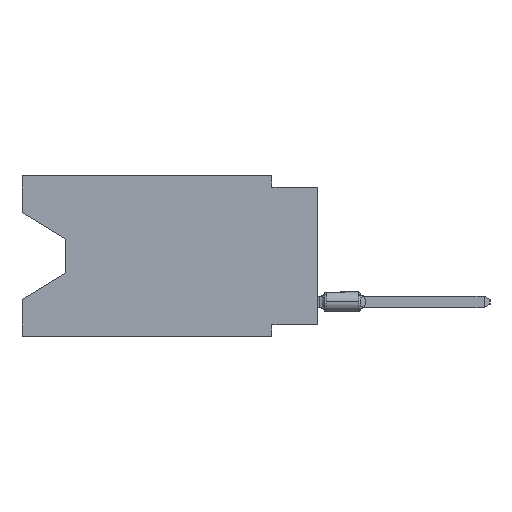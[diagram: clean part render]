
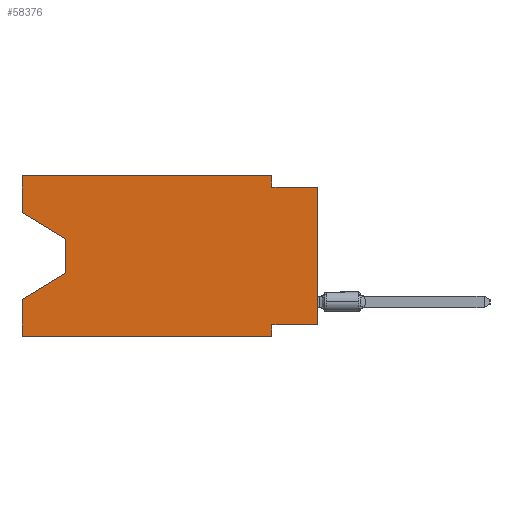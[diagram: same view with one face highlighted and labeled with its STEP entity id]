
A CAD part, left-side view. The second image highlights one B-rep face of the part: STEP entity #58376.
In plain terms, the highlighted planar face has unit normal (-1, 0, 0).
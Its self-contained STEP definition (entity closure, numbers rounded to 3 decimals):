
#305 = ORIENTED_EDGE ( 'NONE', *, *, #55115, .T. ) ;
#1327 = CARTESIAN_POINT ( 'NONE',  ( 0., 2.54, -8.89 ) ) ;
#1581 = DIRECTION ( 'NONE',  ( 0., -1., 0. ) ) ;
#2448 = CARTESIAN_POINT ( 'NONE',  ( 0., 16.383, -6.852 ) ) ;
#2837 = EDGE_CURVE ( 'NONE', #50765, #39058, #23167, .T. ) ;
#4071 = VERTEX_POINT ( 'NONE', #55797 ) ;
#4248 = LINE ( 'NONE', #29562, #50675 ) ;
#7455 = DIRECTION ( 'NONE',  ( 0., -0.855, -0.519 ) ) ;
#7603 = DIRECTION ( 'NONE',  ( 0., -1., 0. ) ) ;
#8316 = EDGE_CURVE ( 'NONE', #63367, #4071, #39837, .T. ) ;
#8692 = CARTESIAN_POINT ( 'NONE',  ( 0., 2.54, -0.635 ) ) ;
#9533 = VECTOR ( 'NONE', #29877, 1000. ) ;
#9950 = ORIENTED_EDGE ( 'NONE', *, *, #14065, .F. ) ;
#11351 = EDGE_CURVE ( 'NONE', #4071, #56030, #33874, .T. ) ;
#11638 = DIRECTION ( 'NONE',  ( 0., 0., 1. ) ) ;
#11701 = DIRECTION ( 'NONE',  ( 0., -1., 0. ) ) ;
#11794 = LINE ( 'NONE', #48024, #45046 ) ;
#12198 = ORIENTED_EDGE ( 'NONE', *, *, #36710, .F. ) ;
#14065 = EDGE_CURVE ( 'NONE', #38638, #59278, #53231, .T. ) ;
#14668 = DIRECTION ( 'NONE',  ( 1., 0., 0. ) ) ;
#14803 = LINE ( 'NONE', #50721, #9533 ) ;
#15726 = VECTOR ( 'NONE', #1581, 1000. ) ;
#16935 = CARTESIAN_POINT ( 'NONE',  ( 0., 2.54, -8.255 ) ) ;
#17046 = ORIENTED_EDGE ( 'NONE', *, *, #34735, .F. ) ;
#17070 = CARTESIAN_POINT ( 'NONE',  ( 0., 16.383, -2.038 ) ) ;
#18257 = VERTEX_POINT ( 'NONE', #30647 ) ;
#19648 = VERTEX_POINT ( 'NONE', #2448 ) ;
#19785 = PLANE ( 'NONE',  #64346 ) ;
#20865 = EDGE_CURVE ( 'NONE', #18257, #19648, #30411, .T. ) ;
#22042 = DIRECTION ( 'NONE',  ( 0., 0., -1. ) ) ;
#22312 = EDGE_LOOP ( 'NONE', ( #29484, #305, #37327, #27753, #54468, #50413, #12198, #62773, #9950, #17046, #22792, #58764 ) ) ;
#22792 = ORIENTED_EDGE ( 'NONE', *, *, #11351, .F. ) ;
#22970 = CARTESIAN_POINT ( 'NONE',  ( 0., 2.54, -8.89 ) ) ;
#23167 = LINE ( 'NONE', #1327, #33071 ) ;
#25918 = VECTOR ( 'NONE', #66521, 1000. ) ;
#26799 = EDGE_CURVE ( 'NONE', #63367, #64253, #28662, .T. ) ;
#27628 = DIRECTION ( 'NONE',  ( 0., 0., -1. ) ) ;
#27659 = VECTOR ( 'NONE', #11638, 1000. ) ;
#27753 = ORIENTED_EDGE ( 'NONE', *, *, #20865, .F. ) ;
#28565 = CARTESIAN_POINT ( 'NONE',  ( 0., 13.97, -3.505 ) ) ;
#28662 = LINE ( 'NONE', #17070, #35437 ) ;
#29390 = DIRECTION ( 'NONE',  ( 0., 0., 1. ) ) ;
#29484 = ORIENTED_EDGE ( 'NONE', *, *, #26799, .T. ) ;
#29562 = CARTESIAN_POINT ( 'NONE',  ( 0., 0., -8.255 ) ) ;
#29877 = DIRECTION ( 'NONE',  ( 0., 0., -1. ) ) ;
#30188 = EDGE_CURVE ( 'NONE', #64141, #59278, #32828, .T. ) ;
#30411 = LINE ( 'NONE', #67000, #44771 ) ;
#30419 = CARTESIAN_POINT ( 'NONE',  ( 0., 13.97, -5.385 ) ) ;
#30647 = CARTESIAN_POINT ( 'NONE',  ( 0., 16.383, -8.89 ) ) ;
#32828 = LINE ( 'NONE', #37625, #27659 ) ;
#33071 = VECTOR ( 'NONE', #49503, 1000. ) ;
#33281 = VECTOR ( 'NONE', #7603, 1000. ) ;
#33874 = LINE ( 'NONE', #59551, #55864 ) ;
#34735 = EDGE_CURVE ( 'NONE', #56030, #38638, #11794, .T. ) ;
#35385 = DIRECTION ( 'NONE',  ( 0., 1., 0. ) ) ;
#35437 = VECTOR ( 'NONE', #7455, 1000. ) ;
#36506 = EDGE_CURVE ( 'NONE', #18257, #39058, #59015, .T. ) ;
#36710 = EDGE_CURVE ( 'NONE', #64141, #50765, #4248, .T. ) ;
#37029 = VECTOR ( 'NONE', #43420, 1000. ) ;
#37327 = ORIENTED_EDGE ( 'NONE', *, *, #52037, .T. ) ;
#37625 = CARTESIAN_POINT ( 'NONE',  ( 0., 0., 0. ) ) ;
#38638 = VERTEX_POINT ( 'NONE', #8692 ) ;
#39058 = VERTEX_POINT ( 'NONE', #22970 ) ;
#39837 = LINE ( 'NONE', #40173, #25918 ) ;
#40173 = CARTESIAN_POINT ( 'NONE',  ( 0., 16.383, 0. ) ) ;
#40987 = FACE_OUTER_BOUND ( 'NONE', #22312, .T. ) ;
#43290 = CARTESIAN_POINT ( 'NONE',  ( 0., 16.383, -8.89 ) ) ;
#43420 = DIRECTION ( 'NONE',  ( 0., 0.855, -0.519 ) ) ;
#44771 = VECTOR ( 'NONE', #29390, 1000. ) ;
#45046 = VECTOR ( 'NONE', #22042, 1000. ) ;
#45323 = VERTEX_POINT ( 'NONE', #30419 ) ;
#48024 = CARTESIAN_POINT ( 'NONE',  ( 0., 2.54, 0. ) ) ;
#49503 = DIRECTION ( 'NONE',  ( 0., 0., -1. ) ) ;
#49918 = CARTESIAN_POINT ( 'NONE',  ( 0., 16.383, -2.038 ) ) ;
#50413 = ORIENTED_EDGE ( 'NONE', *, *, #2837, .F. ) ;
#50675 = VECTOR ( 'NONE', #35385, 1000. ) ;
#50721 = CARTESIAN_POINT ( 'NONE',  ( 0., 13.97, -3.505 ) ) ;
#50765 = VERTEX_POINT ( 'NONE', #16935 ) ;
#52037 = EDGE_CURVE ( 'NONE', #45323, #19648, #55023, .T. ) ;
#53231 = LINE ( 'NONE', #54455, #33281 ) ;
#54455 = CARTESIAN_POINT ( 'NONE',  ( 0., 0., -0.635 ) ) ;
#54468 = ORIENTED_EDGE ( 'NONE', *, *, #36506, .T. ) ;
#55023 = LINE ( 'NONE', #60503, #37029 ) ;
#55115 = EDGE_CURVE ( 'NONE', #64253, #45323, #14803, .T. ) ;
#55797 = CARTESIAN_POINT ( 'NONE',  ( 0., 16.383, 0. ) ) ;
#55864 = VECTOR ( 'NONE', #11701, 1000. ) ;
#56030 = VERTEX_POINT ( 'NONE', #63809 ) ;
#58376 = ADVANCED_FACE ( 'NONE', ( #40987 ), #19785, .F. ) ;
#58381 = CARTESIAN_POINT ( 'NONE',  ( 0., 0., -8.255 ) ) ;
#58764 = ORIENTED_EDGE ( 'NONE', *, *, #8316, .F. ) ;
#59015 = LINE ( 'NONE', #43290, #15726 ) ;
#59278 = VERTEX_POINT ( 'NONE', #62848 ) ;
#59551 = CARTESIAN_POINT ( 'NONE',  ( 0., 16.383, 0. ) ) ;
#60503 = CARTESIAN_POINT ( 'NONE',  ( 0., 13.97, -5.385 ) ) ;
#61524 = CARTESIAN_POINT ( 'NONE',  ( 0., 16.383, 0. ) ) ;
#62773 = ORIENTED_EDGE ( 'NONE', *, *, #30188, .T. ) ;
#62848 = CARTESIAN_POINT ( 'NONE',  ( 0., 0., -0.635 ) ) ;
#63367 = VERTEX_POINT ( 'NONE', #49918 ) ;
#63809 = CARTESIAN_POINT ( 'NONE',  ( 0., 2.54, 0. ) ) ;
#64141 = VERTEX_POINT ( 'NONE', #58381 ) ;
#64253 = VERTEX_POINT ( 'NONE', #28565 ) ;
#64346 = AXIS2_PLACEMENT_3D ( 'NONE', #61524, #14668, #27628 ) ;
#66521 = DIRECTION ( 'NONE',  ( 0., 0., 1. ) ) ;
#67000 = CARTESIAN_POINT ( 'NONE',  ( 0., 16.383, 0. ) ) ;
